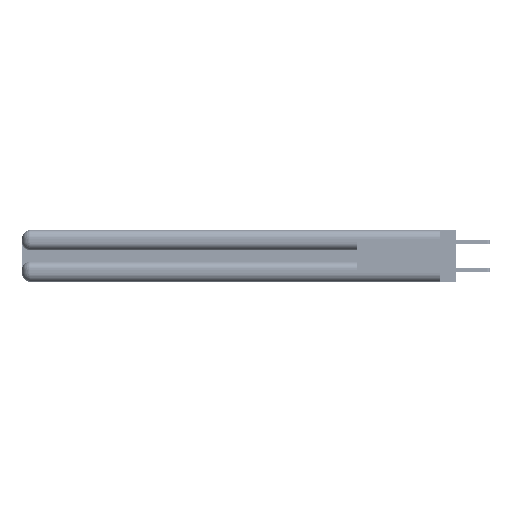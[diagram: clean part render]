
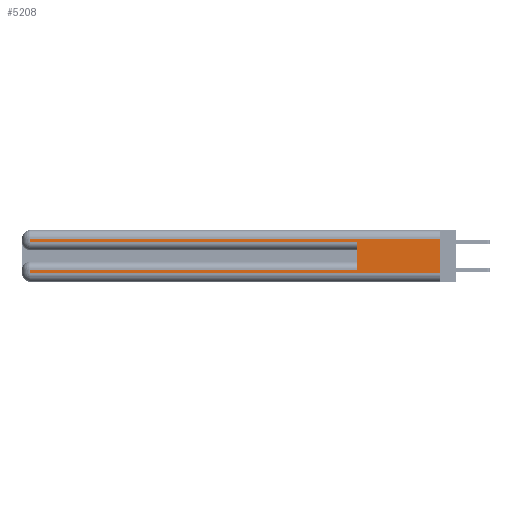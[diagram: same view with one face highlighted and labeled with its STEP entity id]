
A CAD part, left-side view. The second image highlights one B-rep face of the part: STEP entity #5208.
In plain terms, the highlighted planar face has unit normal (-1, 0, 0).
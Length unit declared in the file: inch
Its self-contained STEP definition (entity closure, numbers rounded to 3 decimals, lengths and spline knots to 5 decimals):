
#168 = LINE ( 'NONE', #39599, #37382 ) ;
#597 = DIRECTION ( 'NONE',  ( 0., 1., 0. ) ) ;
#1196 = CARTESIAN_POINT ( 'NONE',  ( 0., 2.94, 0.06 ) ) ;
#1330 = EDGE_CURVE ( 'NONE', #22084, #29757, #168, .T. ) ;
#1738 = CARTESIAN_POINT ( 'NONE',  ( 0., 0.6, 0.085 ) ) ;
#2082 = VECTOR ( 'NONE', #36063, 39.37008 ) ;
#2398 = ORIENTED_EDGE ( 'NONE', *, *, #15355, .T. ) ;
#2639 = VERTEX_POINT ( 'NONE', #6190 ) ;
#2988 = FACE_OUTER_BOUND ( 'NONE', #12174, .T. ) ;
#4109 = VECTOR ( 'NONE', #4474, 39.37008 ) ;
#4474 = DIRECTION ( 'NONE',  ( 0., 0., 1. ) ) ;
#5208 = ADVANCED_FACE ( 'NONE', ( #2988 ), #7287, .F. ) ;
#5405 = LINE ( 'NONE', #9916, #20646 ) ;
#6190 = CARTESIAN_POINT ( 'NONE',  ( 0., 0.6, 0.285 ) ) ;
#6219 = LINE ( 'NONE', #13560, #27728 ) ;
#7287 = PLANE ( 'NONE',  #15198 ) ;
#9879 = LINE ( 'NONE', #37061, #29809 ) ;
#9916 = CARTESIAN_POINT ( 'NONE',  ( 0., 2.94, 0.37 ) ) ;
#10404 = EDGE_CURVE ( 'NONE', #24261, #2639, #9879, .T. ) ;
#10573 = EDGE_CURVE ( 'NONE', #36410, #29470, #6219, .T. ) ;
#11099 = EDGE_CURVE ( 'NONE', #36410, #34215, #12986, .T. ) ;
#11415 = VECTOR ( 'NONE', #597, 39.37008 ) ;
#11785 = VECTOR ( 'NONE', #25225, 39.37008 ) ;
#12174 = EDGE_LOOP ( 'NONE', ( #23661, #23798, #21733, #20071, #19802, #38141, #2398, #22930 ) ) ;
#12986 = LINE ( 'NONE', #26654, #11415 ) ;
#13560 = CARTESIAN_POINT ( 'NONE',  ( 0., 0., 0.37 ) ) ;
#13941 = DIRECTION ( 'NONE',  ( 0., 0., -1. ) ) ;
#14984 = EDGE_CURVE ( 'NONE', #34215, #24261, #20687, .T. ) ;
#15198 = AXIS2_PLACEMENT_3D ( 'NONE', #34057, #18469, #31907 ) ;
#15355 = EDGE_CURVE ( 'NONE', #29757, #37407, #5405, .T. ) ;
#16612 = DIRECTION ( 'NONE',  ( 0., -1., 0. ) ) ;
#16631 = CARTESIAN_POINT ( 'NONE',  ( 0., 2.94, 0.31 ) ) ;
#16774 = LINE ( 'NONE', #38873, #2082 ) ;
#17254 = DIRECTION ( 'NONE',  ( 0., 0., -1. ) ) ;
#18469 = DIRECTION ( 'NONE',  ( 1., 0., 0. ) ) ;
#18559 = CARTESIAN_POINT ( 'NONE',  ( 0., 0., 0.06 ) ) ;
#18872 = EDGE_CURVE ( 'NONE', #37407, #29470, #16774, .T. ) ;
#19802 = ORIENTED_EDGE ( 'NONE', *, *, #29973, .F. ) ;
#20071 = ORIENTED_EDGE ( 'NONE', *, *, #10404, .T. ) ;
#20646 = VECTOR ( 'NONE', #17254, 39.37008 ) ;
#20687 = LINE ( 'NONE', #22000, #11785 ) ;
#21072 = CARTESIAN_POINT ( 'NONE',  ( 0., 2.94, 0.085 ) ) ;
#21733 = ORIENTED_EDGE ( 'NONE', *, *, #14984, .T. ) ;
#21823 = CARTESIAN_POINT ( 'NONE',  ( 0., 0.6, 0.145 ) ) ;
#22000 = CARTESIAN_POINT ( 'NONE',  ( 0., 2.94, 0.37 ) ) ;
#22084 = VERTEX_POINT ( 'NONE', #1738 ) ;
#22930 = ORIENTED_EDGE ( 'NONE', *, *, #18872, .T. ) ;
#23661 = ORIENTED_EDGE ( 'NONE', *, *, #10573, .F. ) ;
#23798 = ORIENTED_EDGE ( 'NONE', *, *, #11099, .T. ) ;
#24261 = VERTEX_POINT ( 'NONE', #43328 ) ;
#25225 = DIRECTION ( 'NONE',  ( 0., 0., -1. ) ) ;
#25987 = CARTESIAN_POINT ( 'NONE',  ( 0., 0., 0.31 ) ) ;
#26654 = CARTESIAN_POINT ( 'NONE',  ( 0., 0., 0.31 ) ) ;
#27728 = VECTOR ( 'NONE', #13941, 39.37008 ) ;
#29470 = VERTEX_POINT ( 'NONE', #18559 ) ;
#29757 = VERTEX_POINT ( 'NONE', #21072 ) ;
#29809 = VECTOR ( 'NONE', #16612, 39.37008 ) ;
#29973 = EDGE_CURVE ( 'NONE', #22084, #2639, #37671, .T. ) ;
#31907 = DIRECTION ( 'NONE',  ( 0., 0., -1. ) ) ;
#34057 = CARTESIAN_POINT ( 'NONE',  ( 0., 0., 0.37 ) ) ;
#34215 = VERTEX_POINT ( 'NONE', #16631 ) ;
#36063 = DIRECTION ( 'NONE',  ( 0., -1., 0. ) ) ;
#36410 = VERTEX_POINT ( 'NONE', #25987 ) ;
#37061 = CARTESIAN_POINT ( 'NONE',  ( 0., 0., 0.285 ) ) ;
#37382 = VECTOR ( 'NONE', #42546, 39.37008 ) ;
#37407 = VERTEX_POINT ( 'NONE', #1196 ) ;
#37671 = LINE ( 'NONE', #21823, #4109 ) ;
#38141 = ORIENTED_EDGE ( 'NONE', *, *, #1330, .T. ) ;
#38873 = CARTESIAN_POINT ( 'NONE',  ( 0., 0., 0.06 ) ) ;
#39599 = CARTESIAN_POINT ( 'NONE',  ( 0., 0., 0.085 ) ) ;
#42546 = DIRECTION ( 'NONE',  ( 0., 1., 0. ) ) ;
#43328 = CARTESIAN_POINT ( 'NONE',  ( 0., 2.94, 0.285 ) ) ;
